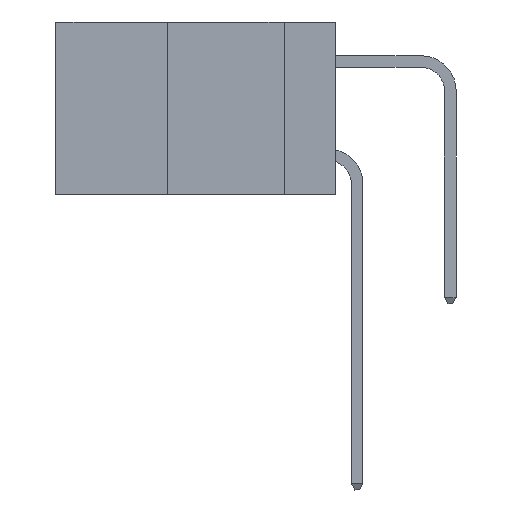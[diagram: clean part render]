
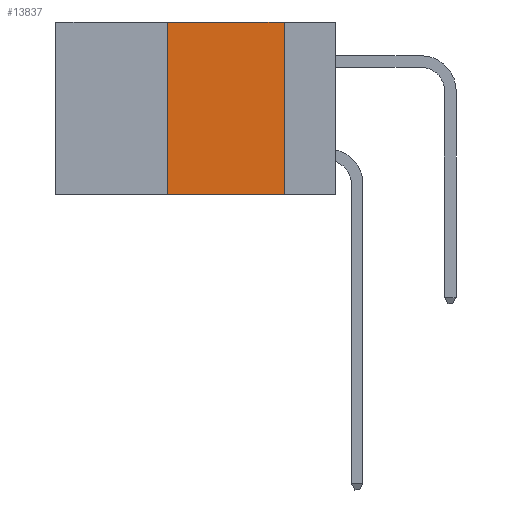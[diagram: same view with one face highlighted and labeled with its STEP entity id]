
A CAD part, left-side view. The second image highlights one B-rep face of the part: STEP entity #13837.
In plain terms, the highlighted planar face has unit normal (-1, 0, 0).
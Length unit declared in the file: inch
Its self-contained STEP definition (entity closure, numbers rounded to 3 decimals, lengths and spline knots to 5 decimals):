
#840 = CARTESIAN_POINT ( 'NONE',  ( 0., 0.11, 0. ) ) ;
#1375 = DIRECTION ( 'NONE',  ( 0., -1., 0. ) ) ;
#5084 = CARTESIAN_POINT ( 'NONE',  ( 0., 0.6, 0. ) ) ;
#5131 = VERTEX_POINT ( 'NONE', #10199 ) ;
#5264 = ORIENTED_EDGE ( 'NONE', *, *, #25988, .F. ) ;
#6855 = LINE ( 'NONE', #5084, #24029 ) ;
#7553 = FACE_OUTER_BOUND ( 'NONE', #28766, .T. ) ;
#8061 = CARTESIAN_POINT ( 'NONE',  ( 0., 0.6, -0.37 ) ) ;
#8806 = EDGE_CURVE ( 'NONE', #5131, #14468, #6855, .T. ) ;
#9494 = DIRECTION ( 'NONE',  ( 0., -1., 0. ) ) ;
#10199 = CARTESIAN_POINT ( 'NONE',  ( 0., 0.36, 0. ) ) ;
#12025 = LINE ( 'NONE', #8061, #13775 ) ;
#13775 = VECTOR ( 'NONE', #1375, 39.37008 ) ;
#13837 = ADVANCED_FACE ( 'NONE', ( #7553 ), #18701, .F. ) ;
#14468 = VERTEX_POINT ( 'NONE', #840 ) ;
#14682 = CARTESIAN_POINT ( 'NONE',  ( 0., 0.36, 0. ) ) ;
#15907 = CARTESIAN_POINT ( 'NONE',  ( 0., 0.11, 0. ) ) ;
#16363 = EDGE_CURVE ( 'NONE', #17716, #28910, #12025, .T. ) ;
#16399 = ORIENTED_EDGE ( 'NONE', *, *, #8806, .F. ) ;
#17191 = CARTESIAN_POINT ( 'NONE',  ( 0., 0.6, 0. ) ) ;
#17716 = VERTEX_POINT ( 'NONE', #28588 ) ;
#18701 = PLANE ( 'NONE',  #27087 ) ;
#18917 = LINE ( 'NONE', #15907, #29083 ) ;
#19546 = DIRECTION ( 'NONE',  ( 1., 0., 0. ) ) ;
#20056 = ORIENTED_EDGE ( 'NONE', *, *, #23520, .F. ) ;
#20227 = VECTOR ( 'NONE', #23538, 39.37008 ) ;
#20937 = ORIENTED_EDGE ( 'NONE', *, *, #16363, .T. ) ;
#22934 = DIRECTION ( 'NONE',  ( 0., 0., -1. ) ) ;
#23520 = EDGE_CURVE ( 'NONE', #17716, #5131, #26160, .T. ) ;
#23538 = DIRECTION ( 'NONE',  ( 0., 0., 1. ) ) ;
#24029 = VECTOR ( 'NONE', #9494, 39.37008 ) ;
#25988 = EDGE_CURVE ( 'NONE', #14468, #28910, #18917, .T. ) ;
#26160 = LINE ( 'NONE', #14682, #20227 ) ;
#26332 = CARTESIAN_POINT ( 'NONE',  ( 0., 0.11, -0.37 ) ) ;
#27087 = AXIS2_PLACEMENT_3D ( 'NONE', #17191, #19546, #28748 ) ;
#28588 = CARTESIAN_POINT ( 'NONE',  ( 0., 0.36, -0.37 ) ) ;
#28748 = DIRECTION ( 'NONE',  ( 0., 0., -1. ) ) ;
#28766 = EDGE_LOOP ( 'NONE', ( #5264, #16399, #20056, #20937 ) ) ;
#28910 = VERTEX_POINT ( 'NONE', #26332 ) ;
#29083 = VECTOR ( 'NONE', #22934, 39.37008 ) ;
